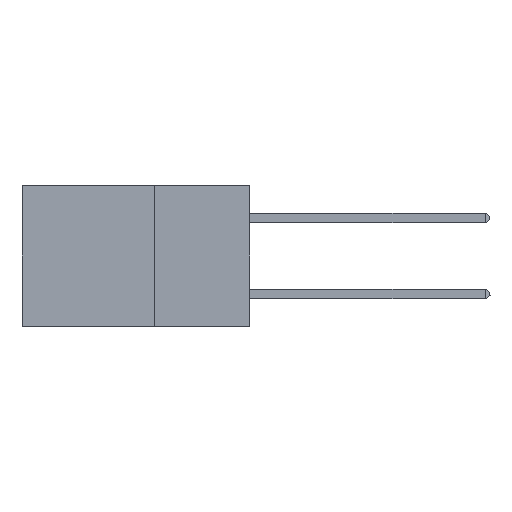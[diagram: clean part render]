
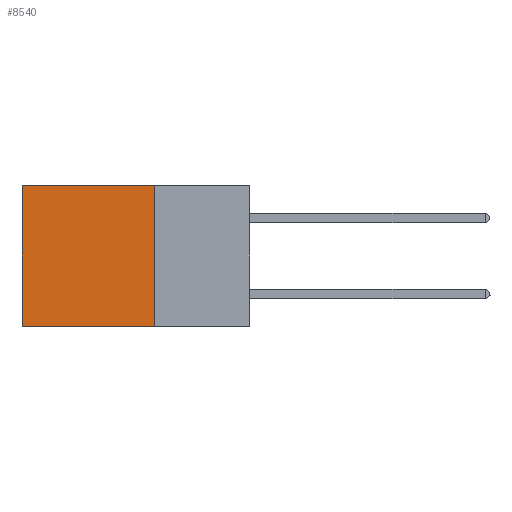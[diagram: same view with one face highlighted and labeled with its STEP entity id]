
A CAD part, left-side view. The second image highlights one B-rep face of the part: STEP entity #8540.
In plain terms, the highlighted planar face has unit normal (-1, 0, 0).
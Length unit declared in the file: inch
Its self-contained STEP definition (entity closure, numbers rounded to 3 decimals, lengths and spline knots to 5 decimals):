
#654 = ORIENTED_EDGE ( 'NONE', *, *, #7939, .T. ) ;
#1426 = EDGE_CURVE ( 'NONE', #5778, #34430, #34527, .T. ) ;
#2144 = VERTEX_POINT ( 'NONE', #22693 ) ;
#2336 = CARTESIAN_POINT ( 'NONE',  ( 0.2875, 0.25, 0. ) ) ;
#2637 = CARTESIAN_POINT ( 'NONE',  ( 0.2875, 0.25, -0.37 ) ) ;
#4088 = ORIENTED_EDGE ( 'NONE', *, *, #11060, .T. ) ;
#5330 = LINE ( 'NONE', #34000, #33809 ) ;
#5778 = VERTEX_POINT ( 'NONE', #17917 ) ;
#7939 = EDGE_CURVE ( 'NONE', #21658, #2144, #5330, .T. ) ;
#8540 = ADVANCED_FACE ( 'NONE', ( #20698 ), #21285, .F. ) ;
#11060 = EDGE_CURVE ( 'NONE', #2144, #34430, #34679, .T. ) ;
#12358 = EDGE_LOOP ( 'NONE', ( #4088, #38426, #14937, #654 ) ) ;
#14763 = DIRECTION ( 'NONE',  ( 0., 0., -1. ) ) ;
#14937 = ORIENTED_EDGE ( 'NONE', *, *, #19470, .F. ) ;
#15708 = DIRECTION ( 'NONE',  ( 0., 0., -1. ) ) ;
#15792 = CARTESIAN_POINT ( 'NONE',  ( 0.2875, 0.25, 0. ) ) ;
#17917 = CARTESIAN_POINT ( 'NONE',  ( 0.2875, 0.25, -0.37 ) ) ;
#19470 = EDGE_CURVE ( 'NONE', #21658, #5778, #40088, .T. ) ;
#20698 = FACE_OUTER_BOUND ( 'NONE', #12358, .T. ) ;
#21285 = PLANE ( 'NONE',  #32805 ) ;
#21658 = VERTEX_POINT ( 'NONE', #15792 ) ;
#22693 = CARTESIAN_POINT ( 'NONE',  ( 0.2875, 0.6, 0. ) ) ;
#24527 = VECTOR ( 'NONE', #28974, 39.37008 ) ;
#27866 = CARTESIAN_POINT ( 'NONE',  ( 0.2875, 0.25, 0. ) ) ;
#28974 = DIRECTION ( 'NONE',  ( 0., 1., 0. ) ) ;
#29582 = VECTOR ( 'NONE', #14763, 39.37008 ) ;
#32697 = VECTOR ( 'NONE', #41272, 39.37008 ) ;
#32805 = AXIS2_PLACEMENT_3D ( 'NONE', #2336, #34982, #15708 ) ;
#33809 = VECTOR ( 'NONE', #36629, 39.37008 ) ;
#34000 = CARTESIAN_POINT ( 'NONE',  ( 0.2875, 0.25, 0. ) ) ;
#34430 = VERTEX_POINT ( 'NONE', #39010 ) ;
#34527 = LINE ( 'NONE', #2637, #24527 ) ;
#34679 = LINE ( 'NONE', #38066, #32697 ) ;
#34982 = DIRECTION ( 'NONE',  ( 1., 0., 0. ) ) ;
#36629 = DIRECTION ( 'NONE',  ( 0., 1., 0. ) ) ;
#38066 = CARTESIAN_POINT ( 'NONE',  ( 0.2875, 0.6, 0. ) ) ;
#38426 = ORIENTED_EDGE ( 'NONE', *, *, #1426, .F. ) ;
#39010 = CARTESIAN_POINT ( 'NONE',  ( 0.2875, 0.6, -0.37 ) ) ;
#40088 = LINE ( 'NONE', #27866, #29582 ) ;
#41272 = DIRECTION ( 'NONE',  ( 0., 0., -1. ) ) ;
